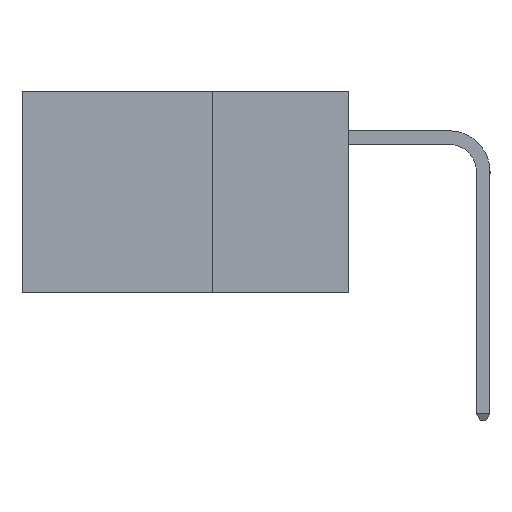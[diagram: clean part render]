
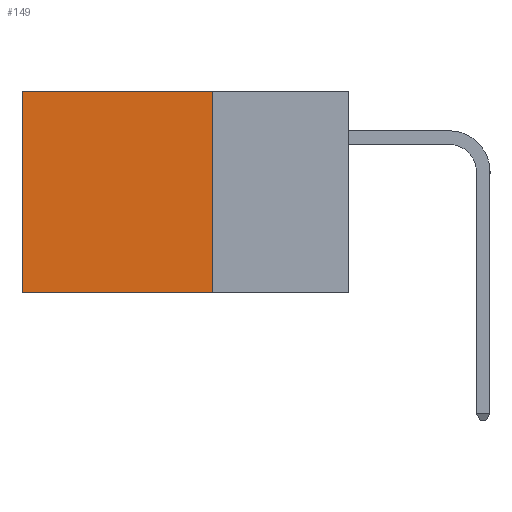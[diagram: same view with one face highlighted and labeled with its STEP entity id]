
A CAD part, left-side view. The second image highlights one B-rep face of the part: STEP entity #149.
In plain terms, the highlighted planar face has unit normal (-1, 0, 0).
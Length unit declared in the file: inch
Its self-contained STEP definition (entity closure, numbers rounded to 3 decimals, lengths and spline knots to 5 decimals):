
#149 = ADVANCED_FACE ( 'NONE', ( #4246 ), #25248, .F. ) ;
#301 = AXIS2_PLACEMENT_3D ( 'NONE', #4110, #13262, #11431 ) ;
#2255 = CARTESIAN_POINT ( 'NONE',  ( 0.2875, 0.6, 0. ) ) ;
#4110 = CARTESIAN_POINT ( 'NONE',  ( 0.2875, 0.25, 0. ) ) ;
#4246 = FACE_OUTER_BOUND ( 'NONE', #24710, .T. ) ;
#4780 = EDGE_CURVE ( 'NONE', #7733, #5168, #11429, .T. ) ;
#5168 = VERTEX_POINT ( 'NONE', #2255 ) ;
#5996 = DIRECTION ( 'NONE',  ( 0., 0., -1. ) ) ;
#6816 = VERTEX_POINT ( 'NONE', #13644 ) ;
#7108 = VECTOR ( 'NONE', #23499, 39.37008 ) ;
#7733 = VERTEX_POINT ( 'NONE', #15962 ) ;
#8523 = CARTESIAN_POINT ( 'NONE',  ( 0.2875, 0.25, 0. ) ) ;
#9299 = CARTESIAN_POINT ( 'NONE',  ( 0.2875, 0.25, -0.37 ) ) ;
#11287 = DIRECTION ( 'NONE',  ( 0., 1., 0. ) ) ;
#11429 = LINE ( 'NONE', #18631, #27509 ) ;
#11431 = DIRECTION ( 'NONE',  ( 0., 0., -1. ) ) ;
#12033 = VERTEX_POINT ( 'NONE', #9299 ) ;
#13007 = ORIENTED_EDGE ( 'NONE', *, *, #4780, .T. ) ;
#13238 = EDGE_CURVE ( 'NONE', #5168, #6816, #28300, .T. ) ;
#13262 = DIRECTION ( 'NONE',  ( 1., 0., 0. ) ) ;
#13644 = CARTESIAN_POINT ( 'NONE',  ( 0.2875, 0.6, -0.37 ) ) ;
#14356 = CARTESIAN_POINT ( 'NONE',  ( 0.2875, 0.6, 0. ) ) ;
#15962 = CARTESIAN_POINT ( 'NONE',  ( 0.2875, 0.25, 0. ) ) ;
#16031 = EDGE_CURVE ( 'NONE', #7733, #12033, #22329, .T. ) ;
#16391 = DIRECTION ( 'NONE',  ( 0., 1., 0. ) ) ;
#18187 = CARTESIAN_POINT ( 'NONE',  ( 0.2875, 0.25, -0.37 ) ) ;
#18435 = ORIENTED_EDGE ( 'NONE', *, *, #16031, .F. ) ;
#18631 = CARTESIAN_POINT ( 'NONE',  ( 0.2875, 0.25, 0. ) ) ;
#19846 = EDGE_CURVE ( 'NONE', #12033, #6816, #27488, .T. ) ;
#22329 = LINE ( 'NONE', #8523, #25045 ) ;
#23499 = DIRECTION ( 'NONE',  ( 0., 0., -1. ) ) ;
#23760 = ORIENTED_EDGE ( 'NONE', *, *, #13238, .T. ) ;
#24710 = EDGE_LOOP ( 'NONE', ( #23760, #27369, #18435, #13007 ) ) ;
#25045 = VECTOR ( 'NONE', #5996, 39.37008 ) ;
#25248 = PLANE ( 'NONE',  #301 ) ;
#27369 = ORIENTED_EDGE ( 'NONE', *, *, #19846, .F. ) ;
#27488 = LINE ( 'NONE', #18187, #27965 ) ;
#27509 = VECTOR ( 'NONE', #16391, 39.37008 ) ;
#27965 = VECTOR ( 'NONE', #11287, 39.37008 ) ;
#28300 = LINE ( 'NONE', #14356, #7108 ) ;
